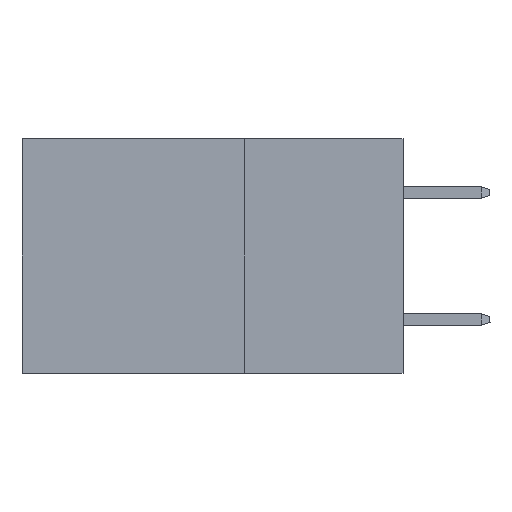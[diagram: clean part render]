
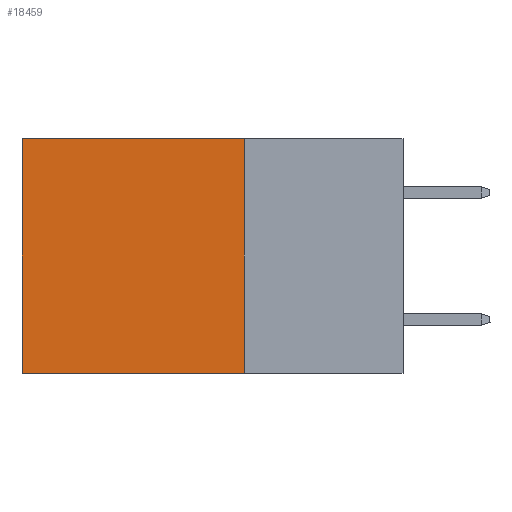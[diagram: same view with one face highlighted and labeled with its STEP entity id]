
A CAD part, left-side view. The second image highlights one B-rep face of the part: STEP entity #18459.
In plain terms, the highlighted planar face has unit normal (-1, 0, 0).
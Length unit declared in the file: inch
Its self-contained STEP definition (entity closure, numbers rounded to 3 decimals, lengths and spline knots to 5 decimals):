
#82 = DIRECTION ( 'NONE',  ( 0., 0., -1. ) ) ;
#2646 = CARTESIAN_POINT ( 'NONE',  ( 0.2875, 0.25, -0.37 ) ) ;
#4814 = DIRECTION ( 'NONE',  ( 0., 0., -1. ) ) ;
#6246 = VERTEX_POINT ( 'NONE', #26803 ) ;
#6266 = DIRECTION ( 'NONE',  ( 0., 1., 0. ) ) ;
#6322 = VECTOR ( 'NONE', #23857, 39.37008 ) ;
#6881 = FACE_OUTER_BOUND ( 'NONE', #7086, .T. ) ;
#7086 = EDGE_LOOP ( 'NONE', ( #17364, #24628, #13320, #8098 ) ) ;
#7635 = EDGE_CURVE ( 'NONE', #21928, #13001, #18866, .T. ) ;
#8098 = ORIENTED_EDGE ( 'NONE', *, *, #7635, .T. ) ;
#9083 = PLANE ( 'NONE',  #10892 ) ;
#9972 = VECTOR ( 'NONE', #22305, 39.37008 ) ;
#10830 = CARTESIAN_POINT ( 'NONE',  ( 0.2875, 0.25, 0. ) ) ;
#10892 = AXIS2_PLACEMENT_3D ( 'NONE', #15239, #23581, #4814 ) ;
#11456 = VERTEX_POINT ( 'NONE', #2646 ) ;
#11897 = LINE ( 'NONE', #18077, #9972 ) ;
#12702 = CARTESIAN_POINT ( 'NONE',  ( 0.2875, 0.25, 0. ) ) ;
#13001 = VERTEX_POINT ( 'NONE', #23454 ) ;
#13320 = ORIENTED_EDGE ( 'NONE', *, *, #27050, .F. ) ;
#14647 = LINE ( 'NONE', #18880, #19430 ) ;
#14729 = VECTOR ( 'NONE', #6266, 39.37008 ) ;
#15239 = CARTESIAN_POINT ( 'NONE',  ( 0.2875, 0.25, 0. ) ) ;
#15821 = EDGE_CURVE ( 'NONE', #11456, #6246, #22071, .T. ) ;
#17364 = ORIENTED_EDGE ( 'NONE', *, *, #17653, .T. ) ;
#17653 = EDGE_CURVE ( 'NONE', #13001, #6246, #11897, .T. ) ;
#18077 = CARTESIAN_POINT ( 'NONE',  ( 0.2875, 0.6, 0. ) ) ;
#18459 = ADVANCED_FACE ( 'NONE', ( #6881 ), #9083, .F. ) ;
#18866 = LINE ( 'NONE', #12702, #14729 ) ;
#18880 = CARTESIAN_POINT ( 'NONE',  ( 0.2875, 0.25, 0. ) ) ;
#19430 = VECTOR ( 'NONE', #82, 39.37008 ) ;
#21928 = VERTEX_POINT ( 'NONE', #10830 ) ;
#22071 = LINE ( 'NONE', #23992, #6322 ) ;
#22305 = DIRECTION ( 'NONE',  ( 0., 0., -1. ) ) ;
#23454 = CARTESIAN_POINT ( 'NONE',  ( 0.2875, 0.6, 0. ) ) ;
#23581 = DIRECTION ( 'NONE',  ( 1., 0., 0. ) ) ;
#23857 = DIRECTION ( 'NONE',  ( 0., 1., 0. ) ) ;
#23992 = CARTESIAN_POINT ( 'NONE',  ( 0.2875, 0.25, -0.37 ) ) ;
#24628 = ORIENTED_EDGE ( 'NONE', *, *, #15821, .F. ) ;
#26803 = CARTESIAN_POINT ( 'NONE',  ( 0.2875, 0.6, -0.37 ) ) ;
#27050 = EDGE_CURVE ( 'NONE', #21928, #11456, #14647, .T. ) ;
